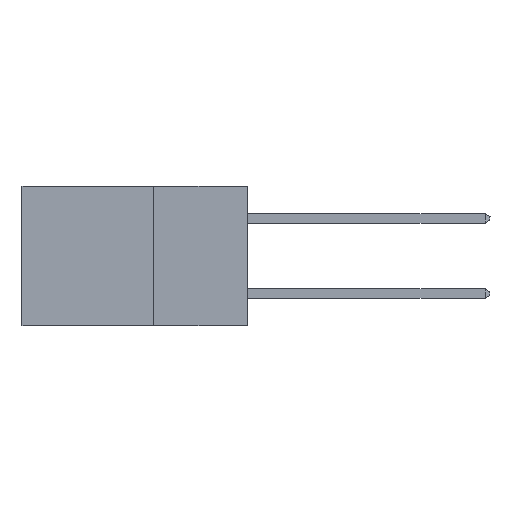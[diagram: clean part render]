
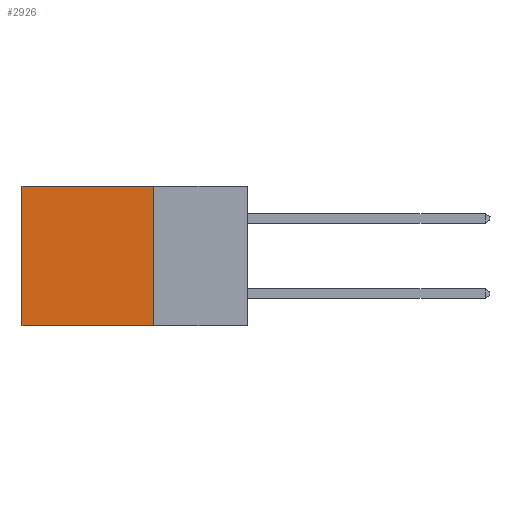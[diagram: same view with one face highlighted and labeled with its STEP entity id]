
A CAD part, left-side view. The second image highlights one B-rep face of the part: STEP entity #2926.
In plain terms, the highlighted planar face has unit normal (-1, 0, 0).
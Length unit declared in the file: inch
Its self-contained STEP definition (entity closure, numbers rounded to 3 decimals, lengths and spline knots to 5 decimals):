
#1287 = AXIS2_PLACEMENT_3D ( 'NONE', #20851, #22350, #22250 ) ;
#2089 = VECTOR ( 'NONE', #22918, 39.37008 ) ;
#2665 = CARTESIAN_POINT ( 'NONE',  ( 0.298, 0.25, 0. ) ) ;
#2832 = LINE ( 'NONE', #20618, #2089 ) ;
#2926 = ADVANCED_FACE ( 'NONE', ( #5358 ), #13981, .F. ) ;
#3271 = LINE ( 'NONE', #2665, #21088 ) ;
#3679 = ORIENTED_EDGE ( 'NONE', *, *, #7141, .T. ) ;
#4425 = CARTESIAN_POINT ( 'NONE',  ( 0.298, 0.25, 0. ) ) ;
#5358 = FACE_OUTER_BOUND ( 'NONE', #5812, .T. ) ;
#5812 = EDGE_LOOP ( 'NONE', ( #3679, #26996, #28137, #25075 ) ) ;
#7141 = EDGE_CURVE ( 'NONE', #23806, #24758, #29834, .T. ) ;
#11367 = VECTOR ( 'NONE', #11764, 39.37008 ) ;
#11764 = DIRECTION ( 'NONE',  ( 0., 0., -1. ) ) ;
#12704 = CARTESIAN_POINT ( 'NONE',  ( 0.298, 0.6, 0. ) ) ;
#12962 = DIRECTION ( 'NONE',  ( 0., 1., 0. ) ) ;
#13373 = EDGE_CURVE ( 'NONE', #29280, #24758, #15063, .T. ) ;
#13981 = PLANE ( 'NONE',  #1287 ) ;
#14375 = VECTOR ( 'NONE', #12962, 39.37008 ) ;
#15063 = LINE ( 'NONE', #17601, #14375 ) ;
#15074 = VERTEX_POINT ( 'NONE', #4425 ) ;
#17399 = CARTESIAN_POINT ( 'NONE',  ( 0.298, 0.6, 0. ) ) ;
#17601 = CARTESIAN_POINT ( 'NONE',  ( 0.298, 0.25, -0.37 ) ) ;
#18349 = EDGE_CURVE ( 'NONE', #15074, #29280, #3271, .T. ) ;
#19439 = EDGE_CURVE ( 'NONE', #15074, #23806, #2832, .T. ) ;
#20618 = CARTESIAN_POINT ( 'NONE',  ( 0.298, 0.25, 0. ) ) ;
#20851 = CARTESIAN_POINT ( 'NONE',  ( 0.298, 0.25, 0. ) ) ;
#21088 = VECTOR ( 'NONE', #21260, 39.37008 ) ;
#21260 = DIRECTION ( 'NONE',  ( 0., 0., -1. ) ) ;
#21261 = CARTESIAN_POINT ( 'NONE',  ( 0.298, 0.25, -0.37 ) ) ;
#22250 = DIRECTION ( 'NONE',  ( 0., 0., -1. ) ) ;
#22350 = DIRECTION ( 'NONE',  ( 1., 0., 0. ) ) ;
#22918 = DIRECTION ( 'NONE',  ( 0., 1., 0. ) ) ;
#23806 = VERTEX_POINT ( 'NONE', #17399 ) ;
#24758 = VERTEX_POINT ( 'NONE', #27656 ) ;
#25075 = ORIENTED_EDGE ( 'NONE', *, *, #19439, .T. ) ;
#26996 = ORIENTED_EDGE ( 'NONE', *, *, #13373, .F. ) ;
#27656 = CARTESIAN_POINT ( 'NONE',  ( 0.298, 0.6, -0.37 ) ) ;
#28137 = ORIENTED_EDGE ( 'NONE', *, *, #18349, .F. ) ;
#29280 = VERTEX_POINT ( 'NONE', #21261 ) ;
#29834 = LINE ( 'NONE', #12704, #11367 ) ;
